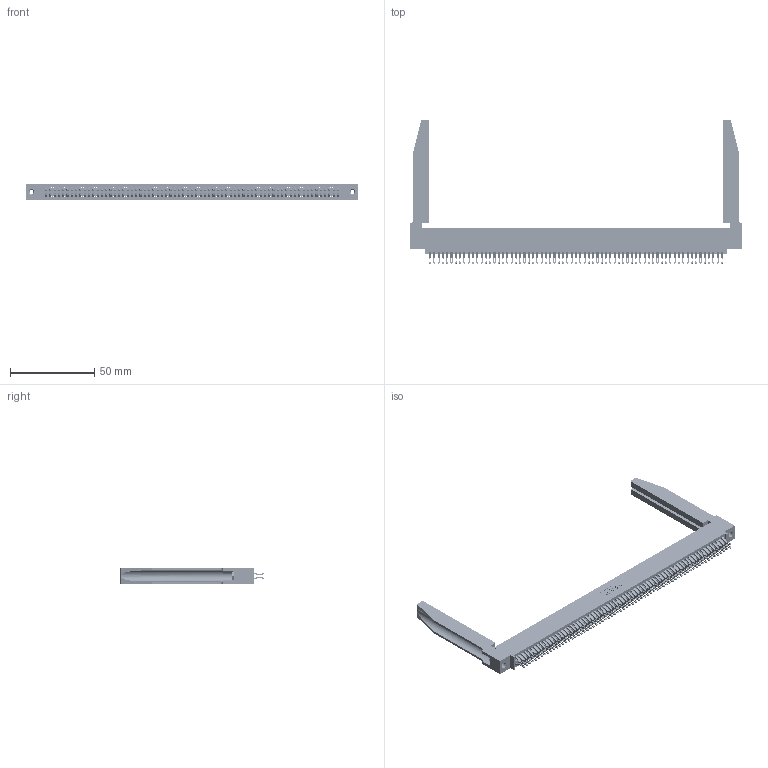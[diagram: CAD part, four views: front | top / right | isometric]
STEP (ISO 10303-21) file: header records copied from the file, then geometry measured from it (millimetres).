
FILE_DESCRIPTION (( 'STEP AP203' ), '1' );
FILE_NAME ('345-138-555-578.STEP', '2019-11-08T16:49:56', ( '' ), ( '' ), 'SwSTEP 2.0', 'SolidWorks 2016', '' );
FILE_SCHEMA (( 'CONFIG_CONTROL_DESIGN' ));
Length unit declared in the file: inch
Products named in the file (5): 345-292-001_555 Tail; 345 Part_0.110 Offset - 0.156 Dia-TH; 345-220-078_345-220-078; 345-138-555-578; 345-250-001_345-250-001-102
Assembly tree (143 placements, depth 2):
  345-138-555-578
    345 Part_0.110 Offset - 0.156 Dia-TH
    345-292-001_555 Tail  x138
    345-250-001_345-250-001-102  x2
    345-220-078_345-220-078  x2
Bounding box: 196.49 x 84.89 x 9.4 mm (x, y, z)
Volume: 27435.6 mm3; surface area: 37914.9 mm2
Topology: 143 solids, 143 shells, 8092 faces, 25387 edges, 16914 vertices
Faces by surface type: plane 4504, cylinder 3536, bspline 36, cone 12, torus 4
Entity records: 55702 total; most frequent: CARTESIAN_POINT 10265, ORIENTED_EDGE 9066, DIRECTION 7979, EDGE_CURVE 4533, VECTOR 4011, LINE 4011, VERTEX_POINT 3016, AXIS2_PLACEMENT_3D 1984
